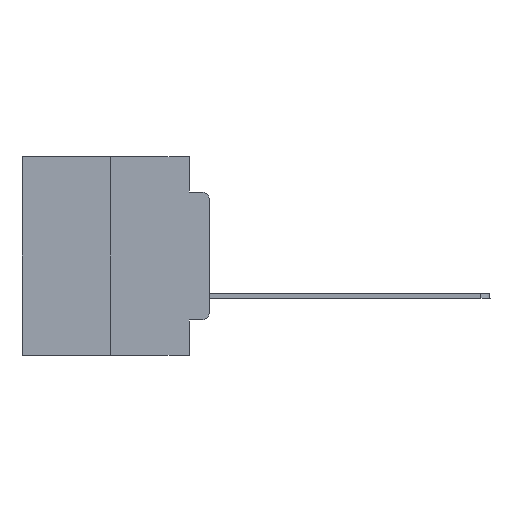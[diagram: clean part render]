
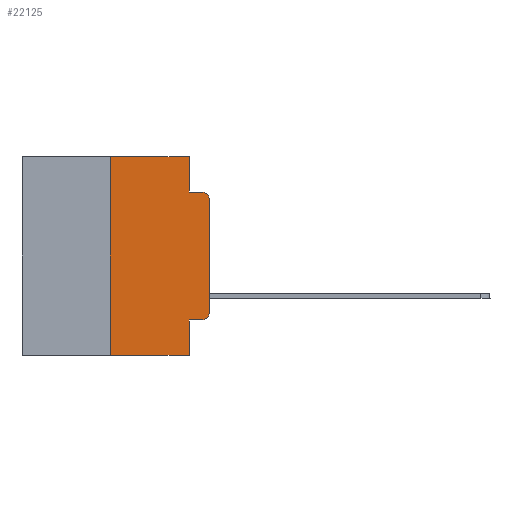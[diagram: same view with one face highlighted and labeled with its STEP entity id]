
A CAD part, left-side view. The second image highlights one B-rep face of the part: STEP entity #22125.
In plain terms, the highlighted planar face has unit normal (-1, 0, 0).
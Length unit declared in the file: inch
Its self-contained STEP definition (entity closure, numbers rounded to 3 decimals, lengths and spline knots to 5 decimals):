
#726 = VERTEX_POINT ( 'NONE', #7906 ) ;
#1190 = EDGE_CURVE ( 'NONE', #3195, #18909, #11867, .T. ) ;
#1587 = EDGE_CURVE ( 'NONE', #12392, #12347, #7948, .T. ) ;
#2149 = ORIENTED_EDGE ( 'NONE', *, *, #1587, .T. ) ;
#3169 = LINE ( 'NONE', #20600, #12588 ) ;
#3195 = VERTEX_POINT ( 'NONE', #4101 ) ;
#3431 = VECTOR ( 'NONE', #9462, 39.37008 ) ;
#3524 = EDGE_CURVE ( 'NONE', #23978, #6502, #3169, .T. ) ;
#3789 = DIRECTION ( 'NONE',  ( 0., 0., 1. ) ) ;
#3804 = DIRECTION ( 'NONE',  ( 1., 0., 0. ) ) ;
#3907 = VERTEX_POINT ( 'NONE', #25938 ) ;
#4054 = EDGE_CURVE ( 'NONE', #3195, #3907, #7655, .T. ) ;
#4101 = CARTESIAN_POINT ( 'NONE',  ( 0., 0.051, -0.4115 ) ) ;
#4660 = VECTOR ( 'NONE', #21691, 39.37008 ) ;
#4771 = CARTESIAN_POINT ( 'NONE',  ( 0., 0.25, 0. ) ) ;
#5960 = LINE ( 'NONE', #6405, #22535 ) ;
#6069 = VECTOR ( 'NONE', #15613, 39.37008 ) ;
#6127 = ORIENTED_EDGE ( 'NONE', *, *, #15873, .T. ) ;
#6270 = ORIENTED_EDGE ( 'NONE', *, *, #3524, .F. ) ;
#6405 = CARTESIAN_POINT ( 'NONE',  ( 0., 0.473, 0. ) ) ;
#6502 = VERTEX_POINT ( 'NONE', #4771 ) ;
#6612 = CARTESIAN_POINT ( 'NONE',  ( 0., 0.051, -0.5 ) ) ;
#6632 = VECTOR ( 'NONE', #14658, 39.37008 ) ;
#7495 = ORIENTED_EDGE ( 'NONE', *, *, #4054, .T. ) ;
#7655 = LINE ( 'NONE', #22661, #20681 ) ;
#7700 = CARTESIAN_POINT ( 'NONE',  ( 0., 0.051, 0. ) ) ;
#7906 = CARTESIAN_POINT ( 'NONE',  ( 0., 0., -0.3915 ) ) ;
#7948 = CIRCLE ( 'NONE', #10437, 0.02 ) ;
#8063 = PLANE ( 'NONE',  #21578 ) ;
#8152 = CARTESIAN_POINT ( 'NONE',  ( 0., 0.051, 0. ) ) ;
#8203 = ORIENTED_EDGE ( 'NONE', *, *, #12714, .F. ) ;
#9462 = DIRECTION ( 'NONE',  ( 0., 0., -1. ) ) ;
#9666 = ORIENTED_EDGE ( 'NONE', *, *, #1190, .F. ) ;
#9676 = CIRCLE ( 'NONE', #14459, 0.02 ) ;
#10011 = CARTESIAN_POINT ( 'NONE',  ( 0., 0.051, 0. ) ) ;
#10437 = AXIS2_PLACEMENT_3D ( 'NONE', #23352, #23174, #23093 ) ;
#11320 = DIRECTION ( 'NONE',  ( -1., 0., 0. ) ) ;
#11813 = CARTESIAN_POINT ( 'NONE',  ( 0., 0.051, -0.0885 ) ) ;
#11867 = LINE ( 'NONE', #7700, #3431 ) ;
#11996 = ORIENTED_EDGE ( 'NONE', *, *, #20892, .F. ) ;
#12187 = LINE ( 'NONE', #24671, #6632 ) ;
#12347 = VERTEX_POINT ( 'NONE', #26021 ) ;
#12392 = VERTEX_POINT ( 'NONE', #19634 ) ;
#12457 = ORIENTED_EDGE ( 'NONE', *, *, #16032, .T. ) ;
#12588 = VECTOR ( 'NONE', #3789, 39.37008 ) ;
#12714 = EDGE_CURVE ( 'NONE', #17583, #19625, #12950, .T. ) ;
#12950 = LINE ( 'NONE', #10011, #17168 ) ;
#13637 = EDGE_CURVE ( 'NONE', #3907, #726, #9676, .T. ) ;
#13773 = CARTESIAN_POINT ( 'NONE',  ( 0., 0.473, -0.5 ) ) ;
#13938 = DIRECTION ( 'NONE',  ( 0., -1., 0. ) ) ;
#14459 = AXIS2_PLACEMENT_3D ( 'NONE', #25157, #11320, #25847 ) ;
#14658 = DIRECTION ( 'NONE',  ( 0., 0., 1. ) ) ;
#15613 = DIRECTION ( 'NONE',  ( 0., -1., 0. ) ) ;
#15873 = EDGE_CURVE ( 'NONE', #726, #12392, #12187, .T. ) ;
#16032 = EDGE_CURVE ( 'NONE', #23978, #18909, #22559, .T. ) ;
#17168 = VECTOR ( 'NONE', #26615, 39.37008 ) ;
#17214 = EDGE_CURVE ( 'NONE', #6502, #17583, #5960, .T. ) ;
#17583 = VERTEX_POINT ( 'NONE', #8152 ) ;
#18345 = ORIENTED_EDGE ( 'NONE', *, *, #17214, .F. ) ;
#18909 = VERTEX_POINT ( 'NONE', #6612 ) ;
#19625 = VERTEX_POINT ( 'NONE', #26089 ) ;
#19634 = CARTESIAN_POINT ( 'NONE',  ( 0., 0., -0.1085 ) ) ;
#19842 = EDGE_LOOP ( 'NONE', ( #6127, #2149, #11996, #8203, #18345, #6270, #12457, #9666, #7495, #22866 ) ) ;
#20600 = CARTESIAN_POINT ( 'NONE',  ( 0., 0.25, 0. ) ) ;
#20681 = VECTOR ( 'NONE', #13938, 39.37008 ) ;
#20892 = EDGE_CURVE ( 'NONE', #19625, #12347, #24610, .T. ) ;
#21578 = AXIS2_PLACEMENT_3D ( 'NONE', #22347, #3804, #24539 ) ;
#21691 = DIRECTION ( 'NONE',  ( 0., -1., 0. ) ) ;
#22125 = ADVANCED_FACE ( 'NONE', ( #26647 ), #8063, .F. ) ;
#22347 = CARTESIAN_POINT ( 'NONE',  ( 0., 0.473, 0. ) ) ;
#22530 = CARTESIAN_POINT ( 'NONE',  ( 0., 0.25, -0.5 ) ) ;
#22535 = VECTOR ( 'NONE', #25041, 39.37008 ) ;
#22559 = LINE ( 'NONE', #13773, #4660 ) ;
#22661 = CARTESIAN_POINT ( 'NONE',  ( 0., 0.051, -0.4115 ) ) ;
#22866 = ORIENTED_EDGE ( 'NONE', *, *, #13637, .T. ) ;
#23093 = DIRECTION ( 'NONE',  ( 0., 0., -1. ) ) ;
#23174 = DIRECTION ( 'NONE',  ( -1., 0., 0. ) ) ;
#23352 = CARTESIAN_POINT ( 'NONE',  ( 0., 0.02, -0.1085 ) ) ;
#23978 = VERTEX_POINT ( 'NONE', #22530 ) ;
#24539 = DIRECTION ( 'NONE',  ( 0., 0., -1. ) ) ;
#24610 = LINE ( 'NONE', #11813, #6069 ) ;
#24671 = CARTESIAN_POINT ( 'NONE',  ( 0., 0., 0. ) ) ;
#25041 = DIRECTION ( 'NONE',  ( 0., -1., 0. ) ) ;
#25157 = CARTESIAN_POINT ( 'NONE',  ( 0., 0.02, -0.3915 ) ) ;
#25847 = DIRECTION ( 'NONE',  ( 0., 0., -1. ) ) ;
#25938 = CARTESIAN_POINT ( 'NONE',  ( 0., 0.02, -0.4115 ) ) ;
#26021 = CARTESIAN_POINT ( 'NONE',  ( 0., 0.02, -0.0885 ) ) ;
#26089 = CARTESIAN_POINT ( 'NONE',  ( 0., 0.051, -0.0885 ) ) ;
#26615 = DIRECTION ( 'NONE',  ( 0., 0., -1. ) ) ;
#26647 = FACE_OUTER_BOUND ( 'NONE', #19842, .T. ) ;
